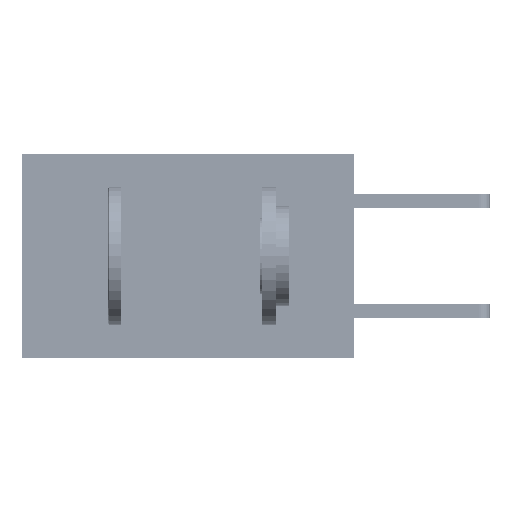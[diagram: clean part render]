
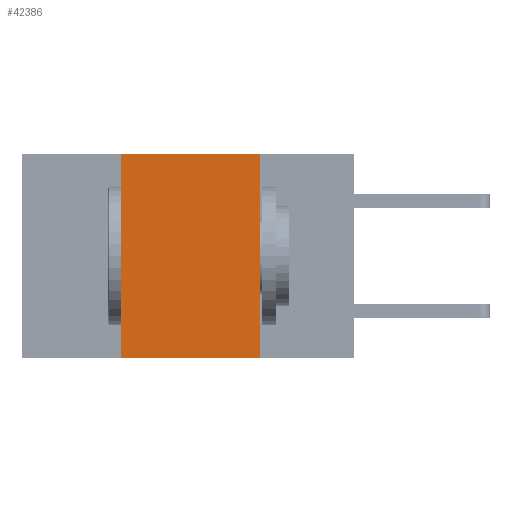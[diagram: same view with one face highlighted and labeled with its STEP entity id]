
A CAD part, left-side view. The second image highlights one B-rep face of the part: STEP entity #42386.
In plain terms, the highlighted planar face has unit normal (-1, 0, 0).
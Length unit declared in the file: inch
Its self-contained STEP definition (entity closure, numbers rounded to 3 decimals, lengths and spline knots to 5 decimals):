
#130 = VECTOR ( 'NONE', #40772, 39.37008 ) ;
#208 = ORIENTED_EDGE ( 'NONE', *, *, #15809, .F. ) ;
#2238 = EDGE_LOOP ( 'NONE', ( #208, #44042, #39700, #23970 ) ) ;
#3241 = CARTESIAN_POINT ( 'NONE',  ( 0., 0.6, 0. ) ) ;
#3353 = CARTESIAN_POINT ( 'NONE',  ( 0., 0.42, 0. ) ) ;
#3651 = VECTOR ( 'NONE', #35637, 39.37008 ) ;
#3765 = CARTESIAN_POINT ( 'NONE',  ( 0., 0.42, -0.37 ) ) ;
#4982 = CARTESIAN_POINT ( 'NONE',  ( 0., 0.42, 0. ) ) ;
#5931 = VECTOR ( 'NONE', #23635, 39.37008 ) ;
#7070 = VERTEX_POINT ( 'NONE', #4982 ) ;
#7178 = CARTESIAN_POINT ( 'NONE',  ( 0., 0.6, -0.37 ) ) ;
#9158 = LINE ( 'NONE', #31654, #43233 ) ;
#13689 = CARTESIAN_POINT ( 'NONE',  ( 0., 0.17, 0. ) ) ;
#14855 = EDGE_CURVE ( 'NONE', #7070, #41835, #31075, .T. ) ;
#15809 = EDGE_CURVE ( 'NONE', #41835, #21219, #9158, .T. ) ;
#17718 = LINE ( 'NONE', #3353, #5931 ) ;
#18689 = DIRECTION ( 'NONE',  ( 0., 0., -1. ) ) ;
#19848 = VERTEX_POINT ( 'NONE', #3765 ) ;
#20939 = DIRECTION ( 'NONE',  ( 1., 0., 0. ) ) ;
#21219 = VERTEX_POINT ( 'NONE', #34950 ) ;
#23635 = DIRECTION ( 'NONE',  ( 0., 0., 1. ) ) ;
#23970 = ORIENTED_EDGE ( 'NONE', *, *, #34472, .T. ) ;
#24364 = CARTESIAN_POINT ( 'NONE',  ( 0., 0.6, 0. ) ) ;
#29859 = DIRECTION ( 'NONE',  ( 0., 0., -1. ) ) ;
#31075 = LINE ( 'NONE', #3241, #130 ) ;
#31654 = CARTESIAN_POINT ( 'NONE',  ( 0., 0.17, 0. ) ) ;
#34265 = AXIS2_PLACEMENT_3D ( 'NONE', #24364, #20939, #29859 ) ;
#34472 = EDGE_CURVE ( 'NONE', #19848, #21219, #40946, .T. ) ;
#34950 = CARTESIAN_POINT ( 'NONE',  ( 0., 0.17, -0.37 ) ) ;
#35637 = DIRECTION ( 'NONE',  ( 0., -1., 0. ) ) ;
#39700 = ORIENTED_EDGE ( 'NONE', *, *, #39782, .F. ) ;
#39782 = EDGE_CURVE ( 'NONE', #19848, #7070, #17718, .T. ) ;
#39864 = FACE_OUTER_BOUND ( 'NONE', #2238, .T. ) ;
#40772 = DIRECTION ( 'NONE',  ( 0., -1., 0. ) ) ;
#40946 = LINE ( 'NONE', #7178, #3651 ) ;
#41027 = PLANE ( 'NONE',  #34265 ) ;
#41835 = VERTEX_POINT ( 'NONE', #13689 ) ;
#42386 = ADVANCED_FACE ( 'NONE', ( #39864 ), #41027, .F. ) ;
#43233 = VECTOR ( 'NONE', #18689, 39.37008 ) ;
#44042 = ORIENTED_EDGE ( 'NONE', *, *, #14855, .F. ) ;
